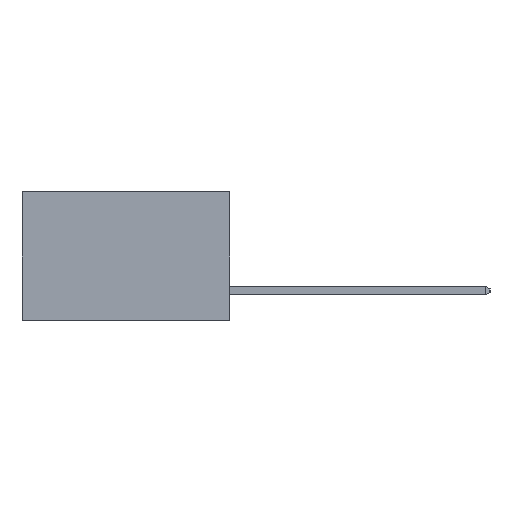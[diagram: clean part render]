
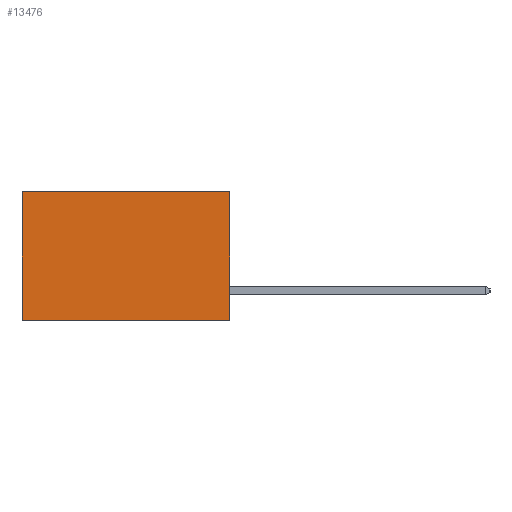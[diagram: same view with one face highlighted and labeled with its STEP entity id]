
A CAD part, left-side view. The second image highlights one B-rep face of the part: STEP entity #13476.
In plain terms, the highlighted planar face has unit normal (-1, 0, 0).
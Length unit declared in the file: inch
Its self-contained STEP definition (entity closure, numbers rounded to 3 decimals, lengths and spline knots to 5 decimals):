
#134 = DIRECTION ( 'NONE',  ( 0., 0., -1. ) ) ;
#169 = CARTESIAN_POINT ( 'NONE',  ( 0.2615, 0., -0.37 ) ) ;
#2110 = VERTEX_POINT ( 'NONE', #8156 ) ;
#2367 = CARTESIAN_POINT ( 'NONE',  ( 0.2615, 0., -0.37 ) ) ;
#2875 = ORIENTED_EDGE ( 'NONE', *, *, #18258, .F. ) ;
#2997 = EDGE_CURVE ( 'NONE', #2110, #5445, #15189, .T. ) ;
#3817 = LINE ( 'NONE', #169, #10858 ) ;
#3913 = LINE ( 'NONE', #2367, #19415 ) ;
#4309 = AXIS2_PLACEMENT_3D ( 'NONE', #10774, #9265, #134 ) ;
#5022 = LINE ( 'NONE', #19178, #12663 ) ;
#5445 = VERTEX_POINT ( 'NONE', #11037 ) ;
#6299 = ORIENTED_EDGE ( 'NONE', *, *, #15369, .T. ) ;
#6917 = DIRECTION ( 'NONE',  ( 0., 1., 0. ) ) ;
#7020 = VECTOR ( 'NONE', #8468, 39.37008 ) ;
#7100 = DIRECTION ( 'NONE',  ( 0., 0., -1. ) ) ;
#8156 = CARTESIAN_POINT ( 'NONE',  ( 0.2615, 0., 0. ) ) ;
#8468 = DIRECTION ( 'NONE',  ( 0., 1., 0. ) ) ;
#8829 = EDGE_LOOP ( 'NONE', ( #6299, #19573, #2875, #12659 ) ) ;
#8889 = VERTEX_POINT ( 'NONE', #13654 ) ;
#9265 = DIRECTION ( 'NONE',  ( 1., 0., 0. ) ) ;
#9853 = CARTESIAN_POINT ( 'NONE',  ( 0.2615, 0., 0. ) ) ;
#10774 = CARTESIAN_POINT ( 'NONE',  ( 0.2615, 0., -0.37 ) ) ;
#10858 = VECTOR ( 'NONE', #15578, 39.37008 ) ;
#10998 = FACE_OUTER_BOUND ( 'NONE', #8829, .T. ) ;
#11037 = CARTESIAN_POINT ( 'NONE',  ( 0.2615, 0.6, 0. ) ) ;
#12379 = PLANE ( 'NONE',  #4309 ) ;
#12659 = ORIENTED_EDGE ( 'NONE', *, *, #2997, .T. ) ;
#12663 = VECTOR ( 'NONE', #7100, 39.37008 ) ;
#13476 = ADVANCED_FACE ( 'NONE', ( #10998 ), #12379, .F. ) ;
#13654 = CARTESIAN_POINT ( 'NONE',  ( 0.2615, 0.6, -0.37 ) ) ;
#14391 = EDGE_CURVE ( 'NONE', #15649, #8889, #3913, .T. ) ;
#15189 = LINE ( 'NONE', #9853, #7020 ) ;
#15369 = EDGE_CURVE ( 'NONE', #5445, #8889, #5022, .T. ) ;
#15578 = DIRECTION ( 'NONE',  ( 0., 0., -1. ) ) ;
#15649 = VERTEX_POINT ( 'NONE', #18227 ) ;
#18227 = CARTESIAN_POINT ( 'NONE',  ( 0.2615, 0., -0.37 ) ) ;
#18258 = EDGE_CURVE ( 'NONE', #2110, #15649, #3817, .T. ) ;
#19178 = CARTESIAN_POINT ( 'NONE',  ( 0.2615, 0.6, -0.37 ) ) ;
#19415 = VECTOR ( 'NONE', #6917, 39.37008 ) ;
#19573 = ORIENTED_EDGE ( 'NONE', *, *, #14391, .F. ) ;
